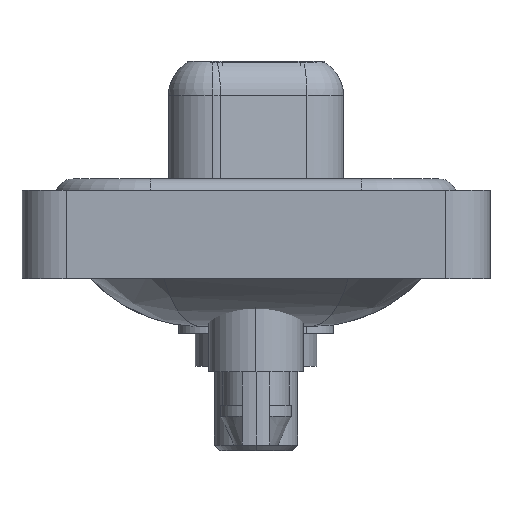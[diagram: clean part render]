
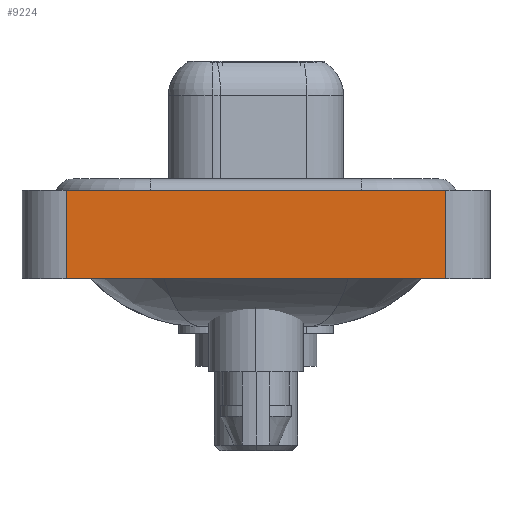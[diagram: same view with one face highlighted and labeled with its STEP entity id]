
A CAD part, left-side view. The second image highlights one B-rep face of the part: STEP entity #9224.
In plain terms, the highlighted planar face has unit normal (-1, 0, 0).
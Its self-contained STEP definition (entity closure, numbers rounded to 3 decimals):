
#211 = VECTOR ( 'NONE', #5717, 1000. ) ;
#1151 = VECTOR ( 'NONE', #6079, 1000. ) ;
#1736 = ORIENTED_EDGE ( 'NONE', *, *, #8263, .F. ) ;
#3084 = VERTEX_POINT ( 'NONE', #14545 ) ;
#3508 = FACE_OUTER_BOUND ( 'NONE', #12428, .T. ) ;
#3825 = PLANE ( 'NONE',  #15881 ) ;
#4397 = CARTESIAN_POINT ( 'NONE',  ( -7.25, -8.55, 0.4 ) ) ;
#4438 = VECTOR ( 'NONE', #15302, 1000. ) ;
#4472 = LINE ( 'NONE', #8068, #211 ) ;
#4823 = LINE ( 'NONE', #6385, #4438 ) ;
#4921 = DIRECTION ( 'NONE',  ( 0., 0., 1. ) ) ;
#5120 = DIRECTION ( 'NONE',  ( 0., -1., 0. ) ) ;
#5717 = DIRECTION ( 'NONE',  ( 0., 0., 1. ) ) ;
#5818 = VERTEX_POINT ( 'NONE', #15993 ) ;
#6079 = DIRECTION ( 'NONE',  ( 0., 0., 1. ) ) ;
#6168 = CARTESIAN_POINT ( 'NONE',  ( -7.25, -8.55, -3.6 ) ) ;
#6385 = CARTESIAN_POINT ( 'NONE',  ( -7.25, -8.55, -3.6 ) ) ;
#6871 = EDGE_CURVE ( 'NONE', #5818, #9569, #4472, .T. ) ;
#7535 = CARTESIAN_POINT ( 'NONE',  ( -7.25, 8.55, 0.4 ) ) ;
#7620 = CARTESIAN_POINT ( 'NONE',  ( -7.25, -8.55, 0.4 ) ) ;
#8068 = CARTESIAN_POINT ( 'NONE',  ( -7.25, -8.55, -3.6 ) ) ;
#8263 = EDGE_CURVE ( 'NONE', #3084, #8931, #16493, .T. ) ;
#8931 = VERTEX_POINT ( 'NONE', #7535 ) ;
#9224 = ADVANCED_FACE ( 'NONE', ( #3508 ), #3825, .T. ) ;
#9569 = VERTEX_POINT ( 'NONE', #4397 ) ;
#9593 = VECTOR ( 'NONE', #5120, 1000. ) ;
#9756 = ORIENTED_EDGE ( 'NONE', *, *, #6871, .T. ) ;
#10213 = EDGE_CURVE ( 'NONE', #8931, #9569, #14865, .T. ) ;
#11293 = DIRECTION ( 'NONE',  ( -1., 0., 0. ) ) ;
#12428 = EDGE_LOOP ( 'NONE', ( #9756, #13093, #1736, #13652 ) ) ;
#12622 = CARTESIAN_POINT ( 'NONE',  ( -7.25, 8.55, -3.6 ) ) ;
#13093 = ORIENTED_EDGE ( 'NONE', *, *, #10213, .F. ) ;
#13652 = ORIENTED_EDGE ( 'NONE', *, *, #15044, .T. ) ;
#14545 = CARTESIAN_POINT ( 'NONE',  ( -7.25, 8.55, -3.6 ) ) ;
#14865 = LINE ( 'NONE', #7620, #9593 ) ;
#15044 = EDGE_CURVE ( 'NONE', #3084, #5818, #4823, .T. ) ;
#15302 = DIRECTION ( 'NONE',  ( 0., -1., 0. ) ) ;
#15881 = AXIS2_PLACEMENT_3D ( 'NONE', #6168, #11293, #4921 ) ;
#15993 = CARTESIAN_POINT ( 'NONE',  ( -7.25, -8.55, -3.6 ) ) ;
#16493 = LINE ( 'NONE', #12622, #1151 ) ;
